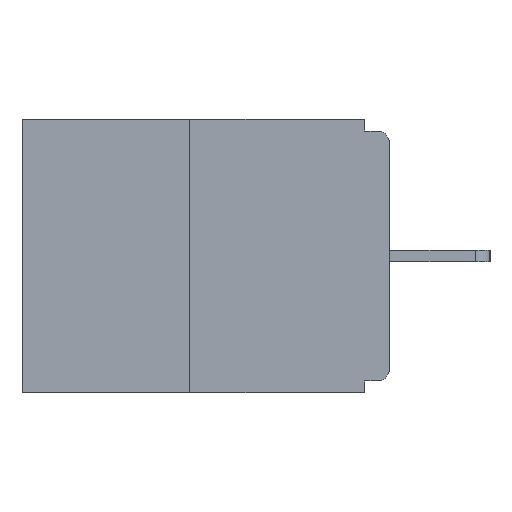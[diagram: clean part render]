
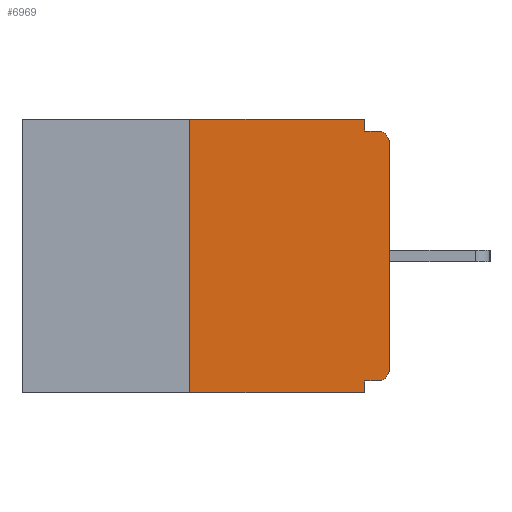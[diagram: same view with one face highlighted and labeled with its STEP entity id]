
A CAD part, left-side view. The second image highlights one B-rep face of the part: STEP entity #6969.
In plain terms, the highlighted planar face has unit normal (-1, 0, 0).
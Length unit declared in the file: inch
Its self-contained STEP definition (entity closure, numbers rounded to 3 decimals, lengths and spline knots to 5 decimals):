
#8 = DIRECTION ( 'NONE',  ( 0., 0., -1. ) ) ;
#473 = VECTOR ( 'NONE', #4655, 39.37008 ) ;
#482 = DIRECTION ( 'NONE',  ( -1., 0., 0. ) ) ;
#612 = AXIS2_PLACEMENT_3D ( 'NONE', #2304, #9297, #3423 ) ;
#731 = EDGE_CURVE ( 'NONE', #5404, #1316, #1724, .T. ) ;
#895 = DIRECTION ( 'NONE',  ( 0., 0., 1. ) ) ;
#932 = CARTESIAN_POINT ( 'NONE',  ( 0., 0.25, 0. ) ) ;
#1316 = VERTEX_POINT ( 'NONE', #8378 ) ;
#1508 = EDGE_CURVE ( 'NONE', #4932, #4132, #7751, .T. ) ;
#1724 = LINE ( 'NONE', #932, #9720 ) ;
#1765 = ORIENTED_EDGE ( 'NONE', *, *, #6122, .F. ) ;
#1871 = PLANE ( 'NONE',  #5104 ) ;
#1986 = CARTESIAN_POINT ( 'NONE',  ( 0., 0., -0.313 ) ) ;
#2109 = CARTESIAN_POINT ( 'NONE',  ( 0., 0., -0.015 ) ) ;
#2304 = CARTESIAN_POINT ( 'NONE',  ( 0., 0.015, -0.313 ) ) ;
#2636 = CARTESIAN_POINT ( 'NONE',  ( 0., 0.46, 0. ) ) ;
#2924 = DIRECTION ( 'NONE',  ( 0., -1., 0. ) ) ;
#2993 = VERTEX_POINT ( 'NONE', #9907 ) ;
#3083 = EDGE_CURVE ( 'NONE', #1316, #4066, #10880, .T. ) ;
#3104 = CARTESIAN_POINT ( 'NONE',  ( 0., 0.031, 0. ) ) ;
#3192 = AXIS2_PLACEMENT_3D ( 'NONE', #6904, #482, #7819 ) ;
#3423 = DIRECTION ( 'NONE',  ( 0., 0., -1. ) ) ;
#3439 = CIRCLE ( 'NONE', #612, 0.015 ) ;
#3578 = DIRECTION ( 'NONE',  ( 0., 0., -1. ) ) ;
#3686 = VECTOR ( 'NONE', #7995, 39.37008 ) ;
#4035 = LINE ( 'NONE', #10747, #3686 ) ;
#4066 = VERTEX_POINT ( 'NONE', #7366 ) ;
#4132 = VERTEX_POINT ( 'NONE', #12860 ) ;
#4511 = VERTEX_POINT ( 'NONE', #1986 ) ;
#4655 = DIRECTION ( 'NONE',  ( 0., -1., 0. ) ) ;
#4726 = VECTOR ( 'NONE', #5357, 39.37008 ) ;
#4733 = EDGE_CURVE ( 'NONE', #4066, #2993, #10408, .T. ) ;
#4767 = VERTEX_POINT ( 'NONE', #5681 ) ;
#4932 = VERTEX_POINT ( 'NONE', #9686 ) ;
#5104 = AXIS2_PLACEMENT_3D ( 'NONE', #9031, #8889, #8878 ) ;
#5136 = CARTESIAN_POINT ( 'NONE',  ( 0., 0.031, -0.343 ) ) ;
#5185 = VECTOR ( 'NONE', #10462, 39.37008 ) ;
#5357 = DIRECTION ( 'NONE',  ( 0., -1., 0. ) ) ;
#5404 = VERTEX_POINT ( 'NONE', #10793 ) ;
#5521 = ORIENTED_EDGE ( 'NONE', *, *, #12001, .T. ) ;
#5681 = CARTESIAN_POINT ( 'NONE',  ( 0., 0., -0.03 ) ) ;
#5981 = CIRCLE ( 'NONE', #3192, 0.015 ) ;
#6122 = EDGE_CURVE ( 'NONE', #2993, #10026, #7357, .T. ) ;
#6289 = EDGE_LOOP ( 'NONE', ( #10076, #6708, #12739, #11345, #12904, #5521, #9179, #6576, #1765, #10894 ) ) ;
#6381 = LINE ( 'NONE', #7971, #11014 ) ;
#6576 = ORIENTED_EDGE ( 'NONE', *, *, #8835, .T. ) ;
#6691 = VERTEX_POINT ( 'NONE', #5136 ) ;
#6708 = ORIENTED_EDGE ( 'NONE', *, *, #731, .F. ) ;
#6904 = CARTESIAN_POINT ( 'NONE',  ( 0., 0.015, -0.03 ) ) ;
#6969 = ADVANCED_FACE ( 'NONE', ( #9624 ), #1871, .F. ) ;
#7116 = CARTESIAN_POINT ( 'NONE',  ( 0., 0., -0.328 ) ) ;
#7357 = LINE ( 'NONE', #2109, #4726 ) ;
#7366 = CARTESIAN_POINT ( 'NONE',  ( 0., 0.031, 0. ) ) ;
#7751 = LINE ( 'NONE', #7116, #5185 ) ;
#7819 = DIRECTION ( 'NONE',  ( 0., 0., -1. ) ) ;
#7971 = CARTESIAN_POINT ( 'NONE',  ( 0., 0.46, -0.343 ) ) ;
#7995 = DIRECTION ( 'NONE',  ( 0., 0., 1. ) ) ;
#8378 = CARTESIAN_POINT ( 'NONE',  ( 0., 0.25, 0. ) ) ;
#8835 = EDGE_CURVE ( 'NONE', #4767, #10026, #5981, .T. ) ;
#8878 = DIRECTION ( 'NONE',  ( 0., 0., -1. ) ) ;
#8889 = DIRECTION ( 'NONE',  ( 1., 0., 0. ) ) ;
#8991 = EDGE_CURVE ( 'NONE', #4511, #4767, #4035, .T. ) ;
#9031 = CARTESIAN_POINT ( 'NONE',  ( 0., 0.46, 0. ) ) ;
#9179 = ORIENTED_EDGE ( 'NONE', *, *, #8991, .T. ) ;
#9211 = EDGE_CURVE ( 'NONE', #4132, #6691, #11223, .T. ) ;
#9297 = DIRECTION ( 'NONE',  ( -1., 0., 0. ) ) ;
#9624 = FACE_OUTER_BOUND ( 'NONE', #6289, .T. ) ;
#9686 = CARTESIAN_POINT ( 'NONE',  ( 0., 0.015, -0.328 ) ) ;
#9720 = VECTOR ( 'NONE', #895, 39.37008 ) ;
#9907 = CARTESIAN_POINT ( 'NONE',  ( 0., 0.031, -0.015 ) ) ;
#10026 = VERTEX_POINT ( 'NONE', #11722 ) ;
#10076 = ORIENTED_EDGE ( 'NONE', *, *, #3083, .F. ) ;
#10408 = LINE ( 'NONE', #3104, #10687 ) ;
#10462 = DIRECTION ( 'NONE',  ( 0., 1., 0. ) ) ;
#10687 = VECTOR ( 'NONE', #3578, 39.37008 ) ;
#10747 = CARTESIAN_POINT ( 'NONE',  ( 0., 0., 0. ) ) ;
#10793 = CARTESIAN_POINT ( 'NONE',  ( 0., 0.25, -0.343 ) ) ;
#10880 = LINE ( 'NONE', #2636, #473 ) ;
#10894 = ORIENTED_EDGE ( 'NONE', *, *, #4733, .F. ) ;
#10925 = VECTOR ( 'NONE', #8, 39.37008 ) ;
#11014 = VECTOR ( 'NONE', #2924, 39.37008 ) ;
#11125 = CARTESIAN_POINT ( 'NONE',  ( 0., 0.031, -0.343 ) ) ;
#11223 = LINE ( 'NONE', #11125, #10925 ) ;
#11345 = ORIENTED_EDGE ( 'NONE', *, *, #9211, .F. ) ;
#11720 = EDGE_CURVE ( 'NONE', #5404, #6691, #6381, .T. ) ;
#11722 = CARTESIAN_POINT ( 'NONE',  ( 0., 0.015, -0.015 ) ) ;
#12001 = EDGE_CURVE ( 'NONE', #4932, #4511, #3439, .T. ) ;
#12739 = ORIENTED_EDGE ( 'NONE', *, *, #11720, .T. ) ;
#12860 = CARTESIAN_POINT ( 'NONE',  ( 0., 0.031, -0.328 ) ) ;
#12904 = ORIENTED_EDGE ( 'NONE', *, *, #1508, .F. ) ;
